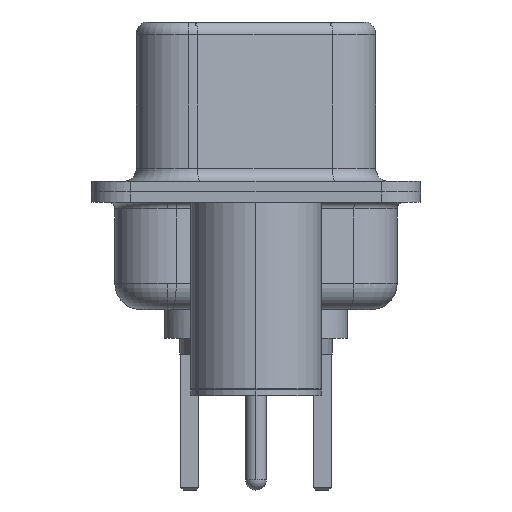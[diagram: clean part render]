
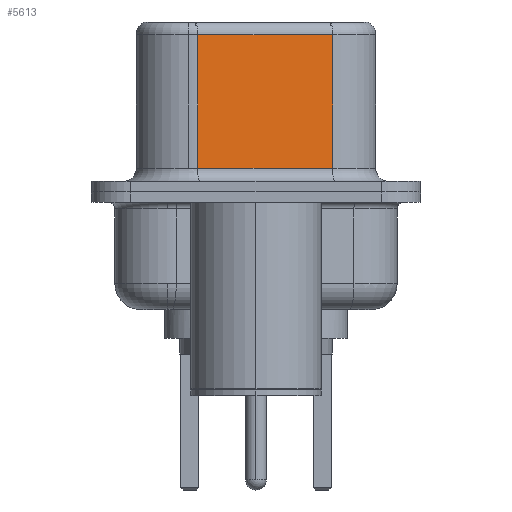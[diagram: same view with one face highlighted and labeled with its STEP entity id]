
A CAD part, left-side view. The second image highlights one B-rep face of the part: STEP entity #5613.
In plain terms, the highlighted planar face has unit normal (-0.985, -0.174, 0).
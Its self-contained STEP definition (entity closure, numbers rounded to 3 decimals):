
#974 = ORIENTED_EDGE ( 'NONE', *, *, #17006, .T. ) ;
#979 = CARTESIAN_POINT ( 'NONE',  ( 3.67, 2.233, 0.9 ) ) ;
#1728 = CARTESIAN_POINT ( 'NONE',  ( 3.67, 2.233, 6.02 ) ) ;
#3846 = CARTESIAN_POINT ( 'NONE',  ( 4.58, -2.927, 6.52 ) ) ;
#3934 = EDGE_CURVE ( 'NONE', #12104, #5176, #18732, .T. ) ;
#3992 = VERTEX_POINT ( 'NONE', #4588 ) ;
#4588 = CARTESIAN_POINT ( 'NONE',  ( 4.58, -2.927, 0.9 ) ) ;
#4947 = CARTESIAN_POINT ( 'NONE',  ( 4.58, -2.927, 6.02 ) ) ;
#5176 = VERTEX_POINT ( 'NONE', #1728 ) ;
#5573 = AXIS2_PLACEMENT_3D ( 'NONE', #3846, #5632, #19599 ) ;
#5613 = ADVANCED_FACE ( 'NONE', ( #22552 ), #17798, .F. ) ;
#5632 = DIRECTION ( 'NONE',  ( 0.985, 0.174, 0. ) ) ;
#7264 = LINE ( 'NONE', #21298, #15509 ) ;
#7359 = VECTOR ( 'NONE', #10749, 1000. ) ;
#8053 = DIRECTION ( 'NONE',  ( 0.174, -0.985, 0. ) ) ;
#9607 = CARTESIAN_POINT ( 'NONE',  ( 4.58, -2.927, 0.9 ) ) ;
#9883 = VERTEX_POINT ( 'NONE', #979 ) ;
#9887 = VECTOR ( 'NONE', #22246, 1000. ) ;
#10217 = ORIENTED_EDGE ( 'NONE', *, *, #21542, .F. ) ;
#10542 = ORIENTED_EDGE ( 'NONE', *, *, #3934, .T. ) ;
#10622 = DIRECTION ( 'NONE',  ( 0., 0., -1. ) ) ;
#10749 = DIRECTION ( 'NONE',  ( 0., 0., -1. ) ) ;
#11449 = EDGE_LOOP ( 'NONE', ( #10217, #10542, #974, #20740 ) ) ;
#12104 = VERTEX_POINT ( 'NONE', #4947 ) ;
#14440 = CARTESIAN_POINT ( 'NONE',  ( 4.58, -2.927, 6.52 ) ) ;
#15509 = VECTOR ( 'NONE', #10622, 1000. ) ;
#16389 = EDGE_CURVE ( 'NONE', #9883, #3992, #16645, .T. ) ;
#16645 = LINE ( 'NONE', #9607, #17194 ) ;
#17006 = EDGE_CURVE ( 'NONE', #5176, #9883, #7264, .T. ) ;
#17194 = VECTOR ( 'NONE', #8053, 1000. ) ;
#17798 = PLANE ( 'NONE',  #5573 ) ;
#17834 = LINE ( 'NONE', #14440, #7359 ) ;
#18732 = LINE ( 'NONE', #20260, #9887 ) ;
#19599 = DIRECTION ( 'NONE',  ( -0.174, 0.985, 0. ) ) ;
#20260 = CARTESIAN_POINT ( 'NONE',  ( 4.58, -2.927, 6.02 ) ) ;
#20740 = ORIENTED_EDGE ( 'NONE', *, *, #16389, .T. ) ;
#21298 = CARTESIAN_POINT ( 'NONE',  ( 3.67, 2.233, 6.52 ) ) ;
#21542 = EDGE_CURVE ( 'NONE', #12104, #3992, #17834, .T. ) ;
#22246 = DIRECTION ( 'NONE',  ( -0.174, 0.985, 0. ) ) ;
#22552 = FACE_OUTER_BOUND ( 'NONE', #11449, .T. ) ;
